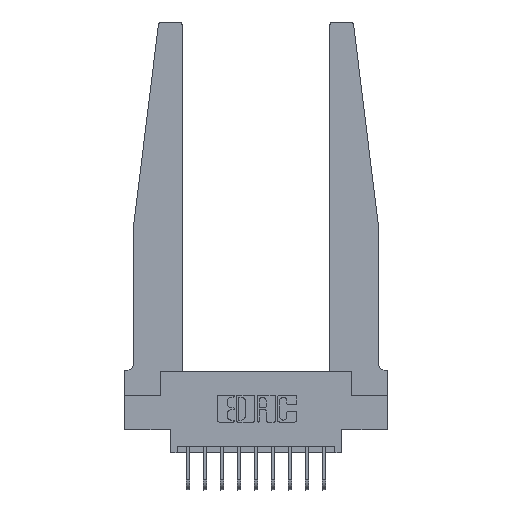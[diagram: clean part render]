
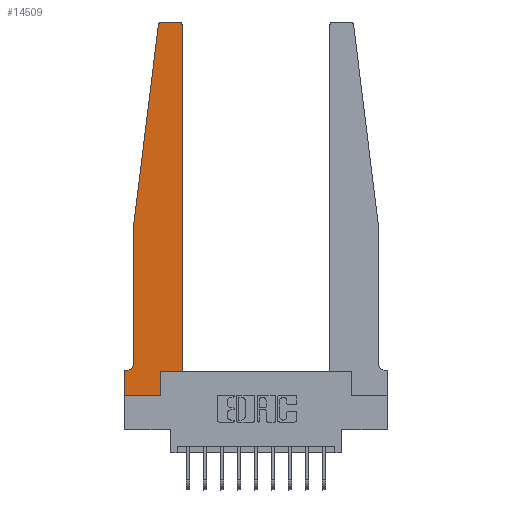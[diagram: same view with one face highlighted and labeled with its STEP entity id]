
A CAD part, top view. The second image highlights one B-rep face of the part: STEP entity #14509.
In plain terms, the highlighted planar face has unit normal (0, 0, 1).
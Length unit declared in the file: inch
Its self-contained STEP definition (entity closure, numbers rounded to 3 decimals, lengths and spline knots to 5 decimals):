
#67 = CARTESIAN_POINT ( 'NONE',  ( 0.27653, 2.72, 0.37 ) ) ;
#85 = LINE ( 'NONE', #161, #1536 ) ;
#154 = LINE ( 'NONE', #1134, #10688 ) ;
#161 = CARTESIAN_POINT ( 'NONE',  ( 0., 0., 0.37 ) ) ;
#190 = ORIENTED_EDGE ( 'NONE', *, *, #9959, .T. ) ;
#229 = EDGE_CURVE ( 'NONE', #17361, #15280, #154, .T. ) ;
#404 = EDGE_CURVE ( 'NONE', #5564, #2871, #7023, .T. ) ;
#748 = VECTOR ( 'NONE', #10213, 39.37008 ) ;
#800 = EDGE_CURVE ( 'NONE', #15280, #3567, #6012, .T. ) ;
#914 = EDGE_CURVE ( 'NONE', #3567, #14498, #14005, .T. ) ;
#963 = DIRECTION ( 'NONE',  ( 0., -1., 0. ) ) ;
#1126 = CARTESIAN_POINT ( 'NONE',  ( 0.395, 2.75, 0.37 ) ) ;
#1134 = CARTESIAN_POINT ( 'NONE',  ( 0.065, 1.25, 0.37 ) ) ;
#1276 = ORIENTED_EDGE ( 'NONE', *, *, #4382, .T. ) ;
#1536 = VECTOR ( 'NONE', #9474, 39.37008 ) ;
#1537 = CARTESIAN_POINT ( 'NONE',  ( 0.425, 0.18, 0.37 ) ) ;
#2418 = ORIENTED_EDGE ( 'NONE', *, *, #914, .T. ) ;
#2871 = VERTEX_POINT ( 'NONE', #12655 ) ;
#2986 = ORIENTED_EDGE ( 'NONE', *, *, #404, .T. ) ;
#3062 = VECTOR ( 'NONE', #16885, 39.37008 ) ;
#3154 = CARTESIAN_POINT ( 'NONE',  ( 0.2605, 0.18, 0.37 ) ) ;
#3251 = EDGE_LOOP ( 'NONE', ( #2986, #1276, #16248, #5761, #2418, #16911, #190, #10532, #16516, #5301, #12720, #13417 ) ) ;
#3268 = CARTESIAN_POINT ( 'NONE',  ( 0.065, 0.2375, 0.37 ) ) ;
#3271 = CARTESIAN_POINT ( 'NONE',  ( 0.425, 0.18, 0.37 ) ) ;
#3567 = VERTEX_POINT ( 'NONE', #3268 ) ;
#3686 = CARTESIAN_POINT ( 'NONE',  ( 0.2605, 0., 0.37 ) ) ;
#3741 = LINE ( 'NONE', #9088, #3062 ) ;
#3948 = VERTEX_POINT ( 'NONE', #16221 ) ;
#4115 = VERTEX_POINT ( 'NONE', #3686 ) ;
#4119 = DIRECTION ( 'NONE',  ( 1., 0., 0. ) ) ;
#4382 = EDGE_CURVE ( 'NONE', #2871, #17361, #12191, .T. ) ;
#5085 = EDGE_CURVE ( 'NONE', #7820, #4115, #8897, .T. ) ;
#5285 = DIRECTION ( 'NONE',  ( -0.122, -0.992, 0. ) ) ;
#5301 = ORIENTED_EDGE ( 'NONE', *, *, #11534, .T. ) ;
#5564 = VERTEX_POINT ( 'NONE', #1126 ) ;
#5761 = ORIENTED_EDGE ( 'NONE', *, *, #800, .T. ) ;
#5784 = DIRECTION ( 'NONE',  ( 0., 1., 0. ) ) ;
#6012 = LINE ( 'NONE', #10138, #13719 ) ;
#6026 = CARTESIAN_POINT ( 'NONE',  ( 0., 0., 0.37 ) ) ;
#6361 = DIRECTION ( 'NONE',  ( 0., 0., 1. ) ) ;
#6388 = VERTEX_POINT ( 'NONE', #12802 ) ;
#6401 = DIRECTION ( 'NONE',  ( 1., 0., 0. ) ) ;
#6718 = AXIS2_PLACEMENT_3D ( 'NONE', #15795, #6361, #15610 ) ;
#6749 = DIRECTION ( 'NONE',  ( 0., 0., 1. ) ) ;
#7023 = LINE ( 'NONE', #9722, #14857 ) ;
#7333 = EDGE_CURVE ( 'NONE', #14498, #3948, #3741, .T. ) ;
#7672 = AXIS2_PLACEMENT_3D ( 'NONE', #67, #16200, #4119 ) ;
#7748 = EDGE_CURVE ( 'NONE', #12598, #5564, #16008, .T. ) ;
#7820 = VERTEX_POINT ( 'NONE', #12255 ) ;
#8127 = DIRECTION ( 'NONE',  ( 0., 1., 0. ) ) ;
#8897 = LINE ( 'NONE', #6026, #17280 ) ;
#9088 = CARTESIAN_POINT ( 'NONE',  ( 0.065, 0.1875, 0.37 ) ) ;
#9180 = VECTOR ( 'NONE', #5784, 39.37008 ) ;
#9273 = LINE ( 'NONE', #12122, #13678 ) ;
#9474 = DIRECTION ( 'NONE',  ( 0., -1., 0. ) ) ;
#9722 = CARTESIAN_POINT ( 'NONE',  ( 0.25, 2.75, 0.37 ) ) ;
#9755 = VERTEX_POINT ( 'NONE', #1537 ) ;
#9959 = EDGE_CURVE ( 'NONE', #3948, #7820, #85, .T. ) ;
#10138 = CARTESIAN_POINT ( 'NONE',  ( 0.065, 1.25, 0.37 ) ) ;
#10213 = DIRECTION ( 'NONE',  ( 1., 0., 0. ) ) ;
#10532 = ORIENTED_EDGE ( 'NONE', *, *, #5085, .T. ) ;
#10534 = CARTESIAN_POINT ( 'NONE',  ( 0., 0.1875, 0.37 ) ) ;
#10688 = VECTOR ( 'NONE', #5285, 39.37008 ) ;
#10815 = EDGE_CURVE ( 'NONE', #9755, #12598, #9273, .T. ) ;
#10844 = CARTESIAN_POINT ( 'NONE',  ( 0.015, 0.2375, 0.37 ) ) ;
#10922 = AXIS2_PLACEMENT_3D ( 'NONE', #10844, #16149, #14823 ) ;
#11079 = CARTESIAN_POINT ( 'NONE',  ( 0.24675, 2.72367, 0.37 ) ) ;
#11534 = EDGE_CURVE ( 'NONE', #6388, #9755, #12769, .T. ) ;
#11680 = EDGE_CURVE ( 'NONE', #4115, #6388, #16539, .T. ) ;
#12039 = CARTESIAN_POINT ( 'NONE',  ( 0.015, 0.1875, 0.37 ) ) ;
#12122 = CARTESIAN_POINT ( 'NONE',  ( 0.425, 0.18, 0.37 ) ) ;
#12191 = CIRCLE ( 'NONE', #7672, 0.03 ) ;
#12255 = CARTESIAN_POINT ( 'NONE',  ( 0., 0., 0.37 ) ) ;
#12598 = VERTEX_POINT ( 'NONE', #14172 ) ;
#12655 = CARTESIAN_POINT ( 'NONE',  ( 0.27653, 2.75, 0.37 ) ) ;
#12720 = ORIENTED_EDGE ( 'NONE', *, *, #10815, .T. ) ;
#12769 = LINE ( 'NONE', #3271, #748 ) ;
#12802 = CARTESIAN_POINT ( 'NONE',  ( 0.2605, 0.18, 0.37 ) ) ;
#13417 = ORIENTED_EDGE ( 'NONE', *, *, #7748, .T. ) ;
#13678 = VECTOR ( 'NONE', #8127, 39.37008 ) ;
#13719 = VECTOR ( 'NONE', #963, 39.37008 ) ;
#14005 = CIRCLE ( 'NONE', #10922, 0.05 ) ;
#14172 = CARTESIAN_POINT ( 'NONE',  ( 0.425, 2.72, 0.37 ) ) ;
#14205 = DIRECTION ( 'NONE',  ( 1., 0., 0. ) ) ;
#14498 = VERTEX_POINT ( 'NONE', #12039 ) ;
#14509 = ADVANCED_FACE ( 'NONE', ( #17434 ), #14601, .T. ) ;
#14601 = PLANE ( 'NONE',  #16278 ) ;
#14823 = DIRECTION ( 'NONE',  ( -1., 0., 0. ) ) ;
#14857 = VECTOR ( 'NONE', #16643, 39.37008 ) ;
#15280 = VERTEX_POINT ( 'NONE', #15941 ) ;
#15610 = DIRECTION ( 'NONE',  ( 1., 0., 0. ) ) ;
#15795 = CARTESIAN_POINT ( 'NONE',  ( 0.395, 2.72, 0.37 ) ) ;
#15941 = CARTESIAN_POINT ( 'NONE',  ( 0.065, 1.25, 0.37 ) ) ;
#16008 = CIRCLE ( 'NONE', #6718, 0.03 ) ;
#16149 = DIRECTION ( 'NONE',  ( 0., 0., -1. ) ) ;
#16200 = DIRECTION ( 'NONE',  ( 0., 0., 1. ) ) ;
#16221 = CARTESIAN_POINT ( 'NONE',  ( 0., 0.1875, 0.37 ) ) ;
#16248 = ORIENTED_EDGE ( 'NONE', *, *, #229, .T. ) ;
#16278 = AXIS2_PLACEMENT_3D ( 'NONE', #10534, #6749, #6401 ) ;
#16516 = ORIENTED_EDGE ( 'NONE', *, *, #11680, .T. ) ;
#16539 = LINE ( 'NONE', #3154, #9180 ) ;
#16643 = DIRECTION ( 'NONE',  ( -1., 0., 0. ) ) ;
#16885 = DIRECTION ( 'NONE',  ( -1., 0., 0. ) ) ;
#16911 = ORIENTED_EDGE ( 'NONE', *, *, #7333, .T. ) ;
#17280 = VECTOR ( 'NONE', #14205, 39.37008 ) ;
#17361 = VERTEX_POINT ( 'NONE', #11079 ) ;
#17434 = FACE_OUTER_BOUND ( 'NONE', #3251, .T. ) ;
